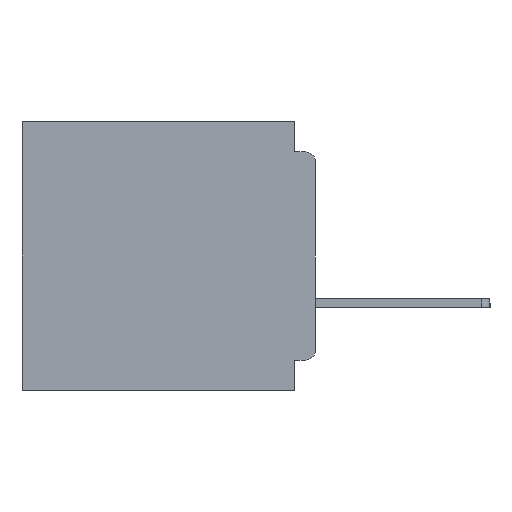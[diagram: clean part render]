
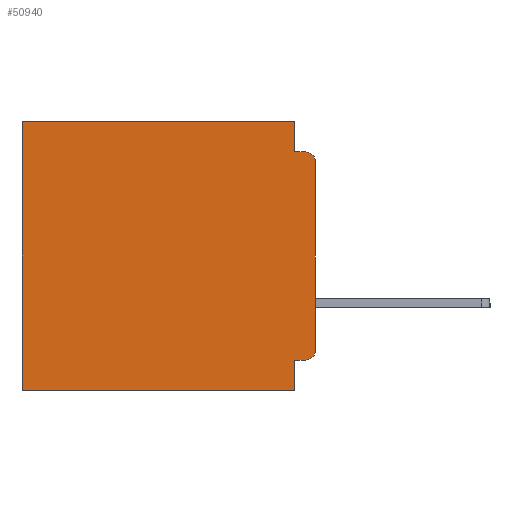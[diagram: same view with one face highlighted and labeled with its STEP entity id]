
A CAD part, left-side view. The second image highlights one B-rep face of the part: STEP entity #50940.
In plain terms, the highlighted planar face has unit normal (-1, 0, 0).
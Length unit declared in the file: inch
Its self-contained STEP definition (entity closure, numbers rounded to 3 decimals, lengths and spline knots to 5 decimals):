
#63 = EDGE_CURVE ( 'NONE', #18980, #37050, #52279, .T. ) ;
#1925 = VECTOR ( 'NONE', #23999, 39.37008 ) ;
#3538 = VECTOR ( 'NONE', #28187, 39.37008 ) ;
#3613 = ORIENTED_EDGE ( 'NONE', *, *, #9912, .T. ) ;
#4246 = ORIENTED_EDGE ( 'NONE', *, *, #23584, .T. ) ;
#6479 = DIRECTION ( 'NONE',  ( 1., 0., 0. ) ) ;
#6909 = CARTESIAN_POINT ( 'NONE',  ( 0.3, 0., -0.355 ) ) ;
#7400 = CARTESIAN_POINT ( 'NONE',  ( 0.3, 0.031, 0. ) ) ;
#8748 = ORIENTED_EDGE ( 'NONE', *, *, #47477, .F. ) ;
#9912 = EDGE_CURVE ( 'NONE', #43205, #25443, #17521, .T. ) ;
#10001 = VERTEX_POINT ( 'NONE', #46202 ) ;
#10410 = EDGE_CURVE ( 'NONE', #41851, #35420, #49828, .T. ) ;
#11717 = CARTESIAN_POINT ( 'NONE',  ( 0.3, 0.031, -0.045 ) ) ;
#12928 = CARTESIAN_POINT ( 'NONE',  ( 0.3, 0.015, -0.045 ) ) ;
#14497 = VECTOR ( 'NONE', #56705, 39.37008 ) ;
#15354 = VERTEX_POINT ( 'NONE', #11717 ) ;
#15526 = EDGE_LOOP ( 'NONE', ( #8748, #23237, #52476, #37127, #48860, #4246, #35488, #23829, #51317, #3613 ) ) ;
#17471 = DIRECTION ( 'NONE',  ( 0., 1., 0. ) ) ;
#17521 = CIRCLE ( 'NONE', #26705, 0.015 ) ;
#18980 = VERTEX_POINT ( 'NONE', #36514 ) ;
#19228 = FACE_OUTER_BOUND ( 'NONE', #15526, .T. ) ;
#19394 = CARTESIAN_POINT ( 'NONE',  ( 0.3, 0.437, -0.4 ) ) ;
#20321 = EDGE_CURVE ( 'NONE', #18980, #15354, #35009, .T. ) ;
#21402 = CARTESIAN_POINT ( 'NONE',  ( 0.3, 0., -0.06 ) ) ;
#21639 = CARTESIAN_POINT ( 'NONE',  ( 0.3, 0.015, -0.06 ) ) ;
#22854 = AXIS2_PLACEMENT_3D ( 'NONE', #21639, #53746, #26250 ) ;
#23237 = ORIENTED_EDGE ( 'NONE', *, *, #45919, .T. ) ;
#23584 = EDGE_CURVE ( 'NONE', #37050, #10001, #25072, .T. ) ;
#23829 = ORIENTED_EDGE ( 'NONE', *, *, #10410, .F. ) ;
#23970 = CARTESIAN_POINT ( 'NONE',  ( 0.3, 0.031, -0.4 ) ) ;
#23999 = DIRECTION ( 'NONE',  ( 0., 0., -1. ) ) ;
#25072 = LINE ( 'NONE', #19394, #1925 ) ;
#25275 = DIRECTION ( 'NONE',  ( 0., 1., 0. ) ) ;
#25443 = VERTEX_POINT ( 'NONE', #34550 ) ;
#25830 = EDGE_CURVE ( 'NONE', #15354, #42043, #49711, .T. ) ;
#26250 = DIRECTION ( 'NONE',  ( 0., 0., -1. ) ) ;
#26705 = AXIS2_PLACEMENT_3D ( 'NONE', #27093, #59089, #31722 ) ;
#26769 = LINE ( 'NONE', #29290, #14497 ) ;
#26830 = LINE ( 'NONE', #52793, #51222 ) ;
#27051 = CARTESIAN_POINT ( 'NONE',  ( 0.3, 0.031, -0.4 ) ) ;
#27093 = CARTESIAN_POINT ( 'NONE',  ( 0.3, 0.015, -0.34 ) ) ;
#27278 = VERTEX_POINT ( 'NONE', #21402 ) ;
#27790 = CARTESIAN_POINT ( 'NONE',  ( 0.3, 0., 0. ) ) ;
#28187 = DIRECTION ( 'NONE',  ( 0., -1., 0. ) ) ;
#29290 = CARTESIAN_POINT ( 'NONE',  ( 0.3, 0., -0.4 ) ) ;
#30183 = DIRECTION ( 'NONE',  ( 0., 1., 0. ) ) ;
#31677 = DIRECTION ( 'NONE',  ( 0., 0., -1. ) ) ;
#31722 = DIRECTION ( 'NONE',  ( 0., 0., -1. ) ) ;
#34208 = CARTESIAN_POINT ( 'NONE',  ( 0.3, 0., -0.4 ) ) ;
#34550 = CARTESIAN_POINT ( 'NONE',  ( 0.3, 0., -0.34 ) ) ;
#35009 = LINE ( 'NONE', #7400, #47152 ) ;
#35420 = VERTEX_POINT ( 'NONE', #23970 ) ;
#35488 = ORIENTED_EDGE ( 'NONE', *, *, #47064, .F. ) ;
#36269 = VECTOR ( 'NONE', #31677, 39.37008 ) ;
#36514 = CARTESIAN_POINT ( 'NONE',  ( 0.3, 0.031, 0. ) ) ;
#37050 = VERTEX_POINT ( 'NONE', #55501 ) ;
#37127 = ORIENTED_EDGE ( 'NONE', *, *, #20321, .F. ) ;
#38872 = DIRECTION ( 'NONE',  ( 0., 0., -1. ) ) ;
#39298 = VECTOR ( 'NONE', #30183, 39.37008 ) ;
#41851 = VERTEX_POINT ( 'NONE', #57278 ) ;
#42043 = VERTEX_POINT ( 'NONE', #12928 ) ;
#42425 = CARTESIAN_POINT ( 'NONE',  ( 0.3, 0.015, -0.355 ) ) ;
#43205 = VERTEX_POINT ( 'NONE', #42425 ) ;
#45187 = EDGE_CURVE ( 'NONE', #43205, #41851, #51372, .T. ) ;
#45919 = EDGE_CURVE ( 'NONE', #27278, #42043, #59196, .T. ) ;
#46202 = CARTESIAN_POINT ( 'NONE',  ( 0.3, 0.437, -0.4 ) ) ;
#47064 = EDGE_CURVE ( 'NONE', #35420, #10001, #26830, .T. ) ;
#47152 = VECTOR ( 'NONE', #48716, 39.37008 ) ;
#47354 = AXIS2_PLACEMENT_3D ( 'NONE', #34208, #6479, #38872 ) ;
#47477 = EDGE_CURVE ( 'NONE', #27278, #25443, #26769, .T. ) ;
#48716 = DIRECTION ( 'NONE',  ( 0., 0., -1. ) ) ;
#48860 = ORIENTED_EDGE ( 'NONE', *, *, #63, .T. ) ;
#49711 = LINE ( 'NONE', #55653, #3538 ) ;
#49828 = LINE ( 'NONE', #27051, #36269 ) ;
#50881 = VECTOR ( 'NONE', #17471, 39.37008 ) ;
#50940 = ADVANCED_FACE ( 'NONE', ( #19228 ), #52382, .F. ) ;
#51222 = VECTOR ( 'NONE', #25275, 39.37008 ) ;
#51317 = ORIENTED_EDGE ( 'NONE', *, *, #45187, .F. ) ;
#51372 = LINE ( 'NONE', #6909, #39298 ) ;
#52279 = LINE ( 'NONE', #27790, #50881 ) ;
#52382 = PLANE ( 'NONE',  #47354 ) ;
#52476 = ORIENTED_EDGE ( 'NONE', *, *, #25830, .F. ) ;
#52793 = CARTESIAN_POINT ( 'NONE',  ( 0.3, 0., -0.4 ) ) ;
#53746 = DIRECTION ( 'NONE',  ( -1., 0., 0. ) ) ;
#55501 = CARTESIAN_POINT ( 'NONE',  ( 0.3, 0.437, 0. ) ) ;
#55653 = CARTESIAN_POINT ( 'NONE',  ( 0.3, 0., -0.045 ) ) ;
#56705 = DIRECTION ( 'NONE',  ( 0., 0., -1. ) ) ;
#57278 = CARTESIAN_POINT ( 'NONE',  ( 0.3, 0.031, -0.355 ) ) ;
#59089 = DIRECTION ( 'NONE',  ( -1., 0., 0. ) ) ;
#59196 = CIRCLE ( 'NONE', #22854, 0.015 ) ;
